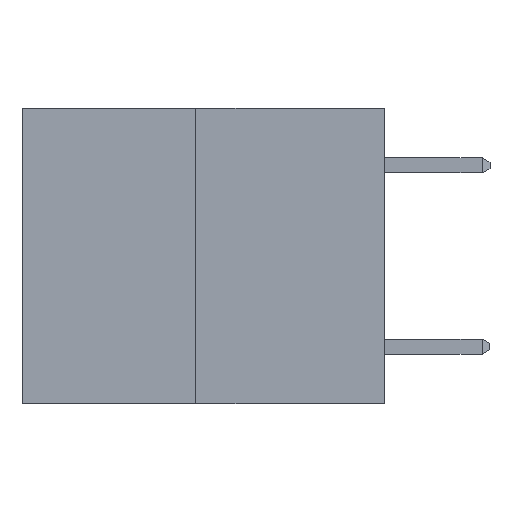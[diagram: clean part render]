
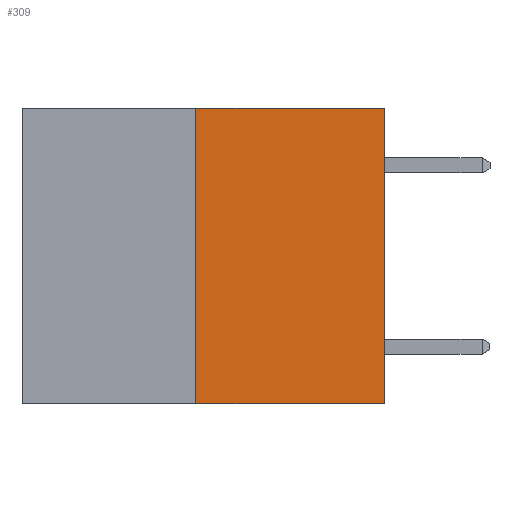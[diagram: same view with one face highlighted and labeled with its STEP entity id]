
A CAD part, left-side view. The second image highlights one B-rep face of the part: STEP entity #309.
In plain terms, the highlighted planar face has unit normal (-1, 0, 0).
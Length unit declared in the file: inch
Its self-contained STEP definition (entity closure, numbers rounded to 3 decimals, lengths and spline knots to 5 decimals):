
#309 = ADVANCED_FACE ( 'NONE', ( #18724 ), #19100, .F. ) ;
#527 = ORIENTED_EDGE ( 'NONE', *, *, #9826, .T. ) ;
#648 = VECTOR ( 'NONE', #2624, 39.37008 ) ;
#894 = AXIS2_PLACEMENT_3D ( 'NONE', #1633, #20400, #17453 ) ;
#1268 = LINE ( 'NONE', #11299, #3259 ) ;
#1633 = CARTESIAN_POINT ( 'NONE',  ( 0., 0.6, 0. ) ) ;
#1753 = VECTOR ( 'NONE', #4108, 39.37008 ) ;
#2624 = DIRECTION ( 'NONE',  ( 0., -1., 0. ) ) ;
#3259 = VECTOR ( 'NONE', #17659, 39.37008 ) ;
#3668 = ORIENTED_EDGE ( 'NONE', *, *, #12297, .T. ) ;
#4108 = DIRECTION ( 'NONE',  ( 0., 0., 1. ) ) ;
#4796 = VERTEX_POINT ( 'NONE', #11734 ) ;
#4873 = LINE ( 'NONE', #8900, #648 ) ;
#4906 = VECTOR ( 'NONE', #15421, 39.37008 ) ;
#6592 = CARTESIAN_POINT ( 'NONE',  ( 0., 0., -0.49 ) ) ;
#7408 = LINE ( 'NONE', #13973, #4906 ) ;
#8110 = EDGE_CURVE ( 'NONE', #9643, #4796, #7408, .T. ) ;
#8900 = CARTESIAN_POINT ( 'NONE',  ( 0., 0.6, -0.49 ) ) ;
#9643 = VERTEX_POINT ( 'NONE', #10706 ) ;
#9722 = VERTEX_POINT ( 'NONE', #6592 ) ;
#9826 = EDGE_CURVE ( 'NONE', #20302, #9722, #4873, .T. ) ;
#10706 = CARTESIAN_POINT ( 'NONE',  ( 0., 0.312, 0. ) ) ;
#11299 = CARTESIAN_POINT ( 'NONE',  ( 0., 0., 0. ) ) ;
#11734 = CARTESIAN_POINT ( 'NONE',  ( 0., 0., 0. ) ) ;
#12046 = CARTESIAN_POINT ( 'NONE',  ( 0., 0.312, -0.49 ) ) ;
#12297 = EDGE_CURVE ( 'NONE', #9722, #4796, #1268, .T. ) ;
#12531 = EDGE_CURVE ( 'NONE', #20302, #9643, #19626, .T. ) ;
#13151 = ORIENTED_EDGE ( 'NONE', *, *, #12531, .F. ) ;
#13973 = CARTESIAN_POINT ( 'NONE',  ( 0., 0.6, 0. ) ) ;
#15421 = DIRECTION ( 'NONE',  ( 0., -1., 0. ) ) ;
#16431 = CARTESIAN_POINT ( 'NONE',  ( 0., 0.312, -0.49 ) ) ;
#17453 = DIRECTION ( 'NONE',  ( 0., 0., -1. ) ) ;
#17659 = DIRECTION ( 'NONE',  ( 0., 0., 1. ) ) ;
#18339 = EDGE_LOOP ( 'NONE', ( #13151, #527, #3668, #19226 ) ) ;
#18724 = FACE_OUTER_BOUND ( 'NONE', #18339, .T. ) ;
#19100 = PLANE ( 'NONE',  #894 ) ;
#19226 = ORIENTED_EDGE ( 'NONE', *, *, #8110, .F. ) ;
#19626 = LINE ( 'NONE', #12046, #1753 ) ;
#20302 = VERTEX_POINT ( 'NONE', #16431 ) ;
#20400 = DIRECTION ( 'NONE',  ( 1., 0., 0. ) ) ;
